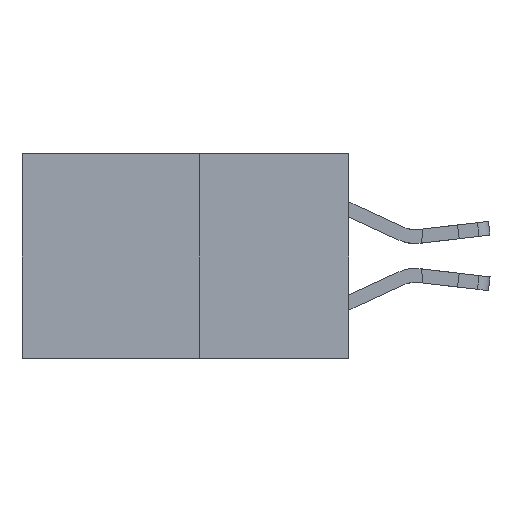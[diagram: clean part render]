
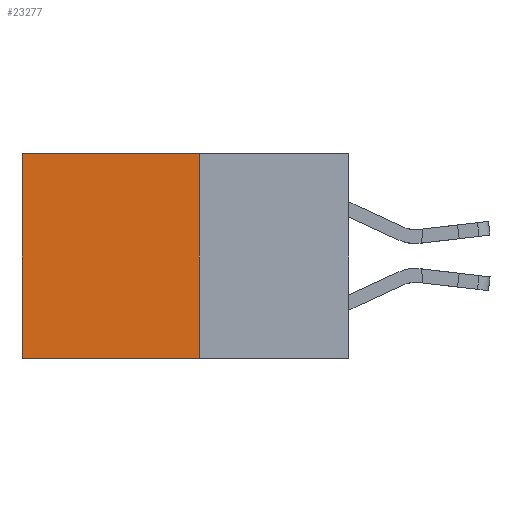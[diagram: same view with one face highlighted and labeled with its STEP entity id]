
A CAD part, left-side view. The second image highlights one B-rep face of the part: STEP entity #23277.
In plain terms, the highlighted planar face has unit normal (-1, 0, 0).
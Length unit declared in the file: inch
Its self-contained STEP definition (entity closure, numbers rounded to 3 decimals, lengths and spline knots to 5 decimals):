
#47 = VERTEX_POINT ( 'NONE', #25630 ) ;
#93 = FACE_OUTER_BOUND ( 'NONE', #3137, .T. ) ;
#1801 = CARTESIAN_POINT ( 'NONE',  ( 0.277, 0.59, -0.37 ) ) ;
#1973 = LINE ( 'NONE', #6460, #19964 ) ;
#2896 = DIRECTION ( 'NONE',  ( 0., 1., 0. ) ) ;
#3137 = EDGE_LOOP ( 'NONE', ( #7125, #15157, #3151, #9117 ) ) ;
#3151 = ORIENTED_EDGE ( 'NONE', *, *, #11062, .F. ) ;
#4715 = EDGE_CURVE ( 'NONE', #16757, #8131, #18457, .T. ) ;
#5694 = LINE ( 'NONE', #6038, #20945 ) ;
#6038 = CARTESIAN_POINT ( 'NONE',  ( 0.277, 0.27, 0. ) ) ;
#6460 = CARTESIAN_POINT ( 'NONE',  ( 0.277, 0.59, -0.37 ) ) ;
#7086 = CARTESIAN_POINT ( 'NONE',  ( 0.277, 0.27, -0.37 ) ) ;
#7125 = ORIENTED_EDGE ( 'NONE', *, *, #23748, .T. ) ;
#7873 = VECTOR ( 'NONE', #2896, 39.37008 ) ;
#8131 = VERTEX_POINT ( 'NONE', #1801 ) ;
#8440 = DIRECTION ( 'NONE',  ( 0., 0., -1. ) ) ;
#8442 = LINE ( 'NONE', #11672, #18418 ) ;
#9060 = PLANE ( 'NONE',  #17458 ) ;
#9117 = ORIENTED_EDGE ( 'NONE', *, *, #16152, .T. ) ;
#9812 = CARTESIAN_POINT ( 'NONE',  ( 0.277, 0.27, -0.37 ) ) ;
#11038 = DIRECTION ( 'NONE',  ( 0., 0., -1. ) ) ;
#11062 = EDGE_CURVE ( 'NONE', #24546, #16757, #8442, .T. ) ;
#11553 = CARTESIAN_POINT ( 'NONE',  ( 0.277, 0.27, 0. ) ) ;
#11672 = CARTESIAN_POINT ( 'NONE',  ( 0.277, 0.27, -0.37 ) ) ;
#13698 = DIRECTION ( 'NONE',  ( 0., 0., -1. ) ) ;
#15157 = ORIENTED_EDGE ( 'NONE', *, *, #4715, .F. ) ;
#16152 = EDGE_CURVE ( 'NONE', #24546, #47, #5694, .T. ) ;
#16462 = CARTESIAN_POINT ( 'NONE',  ( 0.277, 0.27, -0.37 ) ) ;
#16757 = VERTEX_POINT ( 'NONE', #9812 ) ;
#17458 = AXIS2_PLACEMENT_3D ( 'NONE', #7086, #22990, #11038 ) ;
#17962 = DIRECTION ( 'NONE',  ( 0., 1., 0. ) ) ;
#18418 = VECTOR ( 'NONE', #13698, 39.37008 ) ;
#18457 = LINE ( 'NONE', #16462, #7873 ) ;
#19964 = VECTOR ( 'NONE', #8440, 39.37008 ) ;
#20945 = VECTOR ( 'NONE', #17962, 39.37008 ) ;
#22990 = DIRECTION ( 'NONE',  ( 1., 0., 0. ) ) ;
#23277 = ADVANCED_FACE ( 'NONE', ( #93 ), #9060, .F. ) ;
#23748 = EDGE_CURVE ( 'NONE', #47, #8131, #1973, .T. ) ;
#24546 = VERTEX_POINT ( 'NONE', #11553 ) ;
#25630 = CARTESIAN_POINT ( 'NONE',  ( 0.277, 0.59, 0. ) ) ;
